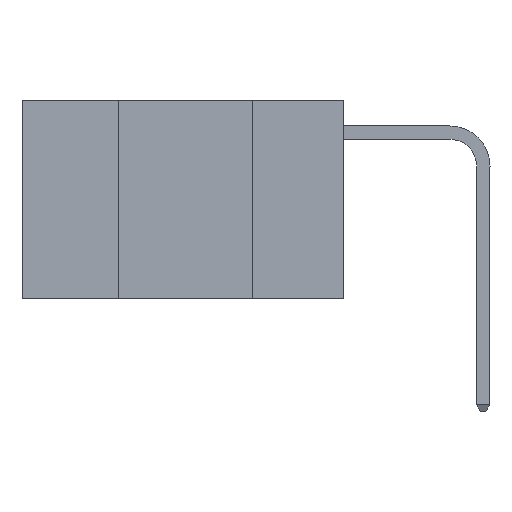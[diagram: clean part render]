
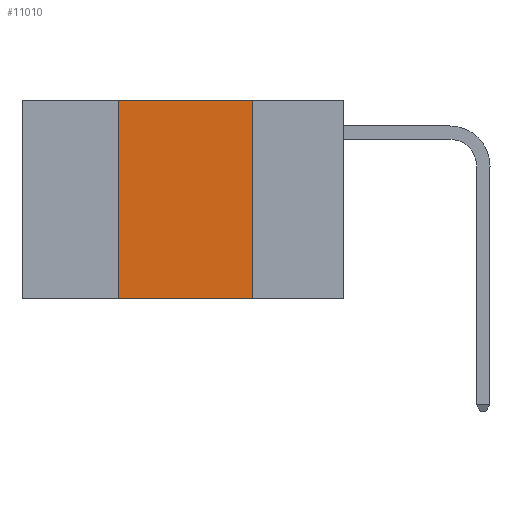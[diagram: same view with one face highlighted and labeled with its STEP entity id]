
A CAD part, left-side view. The second image highlights one B-rep face of the part: STEP entity #11010.
In plain terms, the highlighted planar face has unit normal (-1, 0, 0).
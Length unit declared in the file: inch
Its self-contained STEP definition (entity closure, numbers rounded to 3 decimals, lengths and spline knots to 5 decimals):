
#190 = EDGE_CURVE ( 'NONE', #11349, #5444, #14454, .T. ) ;
#799 = ORIENTED_EDGE ( 'NONE', *, *, #190, .F. ) ;
#1220 = VECTOR ( 'NONE', #6072, 39.37008 ) ;
#2818 = CARTESIAN_POINT ( 'NONE',  ( 0., 0.17, -0.37 ) ) ;
#3145 = DIRECTION ( 'NONE',  ( 0., -1., 0. ) ) ;
#3588 = VECTOR ( 'NONE', #10670, 39.37008 ) ;
#3699 = VERTEX_POINT ( 'NONE', #15373 ) ;
#4695 = CARTESIAN_POINT ( 'NONE',  ( 0., 0.6, 0. ) ) ;
#4882 = CARTESIAN_POINT ( 'NONE',  ( 0., 0.42, 0. ) ) ;
#4911 = LINE ( 'NONE', #4695, #1220 ) ;
#5194 = LINE ( 'NONE', #4882, #5616 ) ;
#5444 = VERTEX_POINT ( 'NONE', #2818 ) ;
#5616 = VECTOR ( 'NONE', #14385, 39.37008 ) ;
#5745 = EDGE_CURVE ( 'NONE', #14208, #3699, #5194, .T. ) ;
#6072 = DIRECTION ( 'NONE',  ( 0., -1., 0. ) ) ;
#6384 = DIRECTION ( 'NONE',  ( 1., 0., 0. ) ) ;
#7679 = PLANE ( 'NONE',  #17076 ) ;
#8142 = VECTOR ( 'NONE', #3145, 39.37008 ) ;
#9979 = CARTESIAN_POINT ( 'NONE',  ( 0., 0.6, -0.37 ) ) ;
#10670 = DIRECTION ( 'NONE',  ( 0., 0., -1. ) ) ;
#11010 = ADVANCED_FACE ( 'NONE', ( #17433 ), #7679, .F. ) ;
#11349 = VERTEX_POINT ( 'NONE', #13814 ) ;
#13571 = EDGE_CURVE ( 'NONE', #14208, #5444, #14981, .T. ) ;
#13814 = CARTESIAN_POINT ( 'NONE',  ( 0., 0.17, 0. ) ) ;
#14208 = VERTEX_POINT ( 'NONE', #15330 ) ;
#14385 = DIRECTION ( 'NONE',  ( 0., 0., 1. ) ) ;
#14454 = LINE ( 'NONE', #14951, #3588 ) ;
#14532 = CARTESIAN_POINT ( 'NONE',  ( 0., 0.6, 0. ) ) ;
#14843 = EDGE_CURVE ( 'NONE', #3699, #11349, #4911, .T. ) ;
#14951 = CARTESIAN_POINT ( 'NONE',  ( 0., 0.17, 0. ) ) ;
#14981 = LINE ( 'NONE', #9979, #8142 ) ;
#15226 = ORIENTED_EDGE ( 'NONE', *, *, #5745, .F. ) ;
#15330 = CARTESIAN_POINT ( 'NONE',  ( 0., 0.42, -0.37 ) ) ;
#15373 = CARTESIAN_POINT ( 'NONE',  ( 0., 0.42, 0. ) ) ;
#15946 = DIRECTION ( 'NONE',  ( 0., 0., -1. ) ) ;
#16000 = EDGE_LOOP ( 'NONE', ( #799, #17192, #15226, #17523 ) ) ;
#17076 = AXIS2_PLACEMENT_3D ( 'NONE', #14532, #6384, #15946 ) ;
#17192 = ORIENTED_EDGE ( 'NONE', *, *, #14843, .F. ) ;
#17433 = FACE_OUTER_BOUND ( 'NONE', #16000, .T. ) ;
#17523 = ORIENTED_EDGE ( 'NONE', *, *, #13571, .T. ) ;
